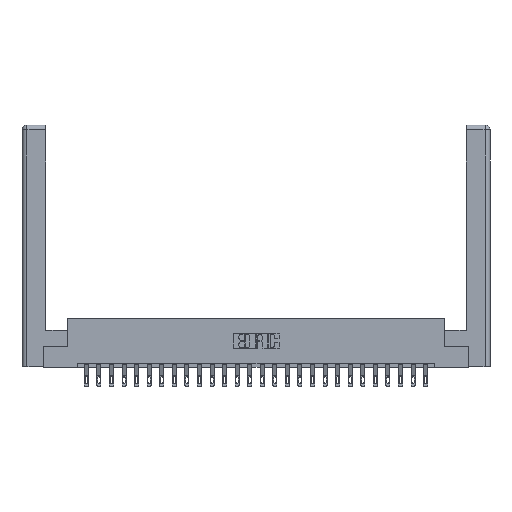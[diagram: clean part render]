
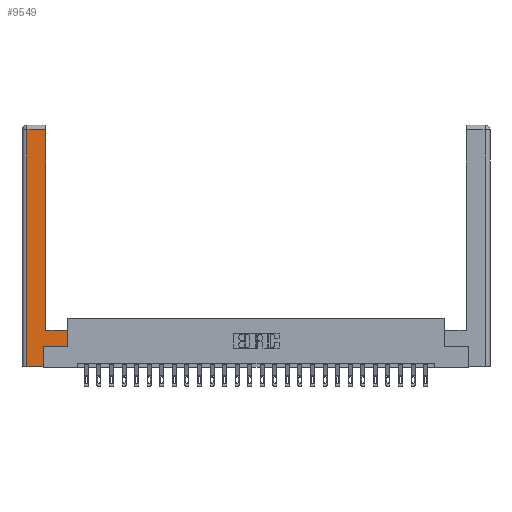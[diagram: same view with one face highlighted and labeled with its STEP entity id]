
A CAD part, top view. The second image highlights one B-rep face of the part: STEP entity #9549.
In plain terms, the highlighted planar face has unit normal (0, 0, 1).
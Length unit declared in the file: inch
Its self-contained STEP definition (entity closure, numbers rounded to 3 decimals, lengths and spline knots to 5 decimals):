
#524 = VECTOR ( 'NONE', #18206, 39.37008 ) ;
#1077 = CARTESIAN_POINT ( 'NONE',  ( 0.295, 0.45, 0. ) ) ;
#1786 = VERTEX_POINT ( 'NONE', #4299 ) ;
#1950 = VECTOR ( 'NONE', #4776, 39.37008 ) ;
#1952 = LINE ( 'NONE', #15213, #2944 ) ;
#2944 = VECTOR ( 'NONE', #9222, 39.37008 ) ;
#3735 = DIRECTION ( 'NONE',  ( 0., -1., 0. ) ) ;
#3939 = DIRECTION ( 'NONE',  ( -1., 0., 0. ) ) ;
#4116 = LINE ( 'NONE', #19426, #13725 ) ;
#4267 = ORIENTED_EDGE ( 'NONE', *, *, #15548, .T. ) ;
#4299 = CARTESIAN_POINT ( 'NONE',  ( 0.0615, 0., 0. ) ) ;
#4776 = DIRECTION ( 'NONE',  ( 0., 1., 0. ) ) ;
#5395 = LINE ( 'NONE', #19114, #13722 ) ;
#6811 = VERTEX_POINT ( 'NONE', #16730 ) ;
#7710 = DIRECTION ( 'NONE',  ( -1., 0., 0. ) ) ;
#8630 = EDGE_CURVE ( 'NONE', #1786, #24178, #4116, .T. ) ;
#8959 = CARTESIAN_POINT ( 'NONE',  ( 0.295, 3., 0. ) ) ;
#9195 = CARTESIAN_POINT ( 'NONE',  ( 0.565, 0.245, 0. ) ) ;
#9222 = DIRECTION ( 'NONE',  ( 1., 0., 0. ) ) ;
#9431 = ORIENTED_EDGE ( 'NONE', *, *, #19889, .T. ) ;
#9549 = ADVANCED_FACE ( 'NONE', ( #22116 ), #11859, .F. ) ;
#9578 = LINE ( 'NONE', #9770, #13397 ) ;
#9770 = CARTESIAN_POINT ( 'NONE',  ( 0.0615, 0., 0. ) ) ;
#10397 = AXIS2_PLACEMENT_3D ( 'NONE', #17906, #26095, #13889 ) ;
#10983 = LINE ( 'NONE', #21126, #1950 ) ;
#11367 = DIRECTION ( 'NONE',  ( 1., 0., 0. ) ) ;
#11859 = PLANE ( 'NONE',  #10397 ) ;
#11881 = EDGE_LOOP ( 'NONE', ( #12309, #22822, #21513, #19605, #4267, #16017, #9431, #15702 ) ) ;
#12309 = ORIENTED_EDGE ( 'NONE', *, *, #19631, .T. ) ;
#12325 = EDGE_CURVE ( 'NONE', #19669, #20694, #1952, .T. ) ;
#13099 = VECTOR ( 'NONE', #3939, 39.37008 ) ;
#13397 = VECTOR ( 'NONE', #3735, 39.37008 ) ;
#13579 = CARTESIAN_POINT ( 'NONE',  ( 0.265, 0.245, 0. ) ) ;
#13644 = EDGE_CURVE ( 'NONE', #21884, #15916, #5395, .T. ) ;
#13722 = VECTOR ( 'NONE', #7710, 39.37008 ) ;
#13725 = VECTOR ( 'NONE', #11367, 39.37008 ) ;
#13889 = DIRECTION ( 'NONE',  ( -1., 0., 0. ) ) ;
#14695 = CARTESIAN_POINT ( 'NONE',  ( 0.0615, 2.94, 0. ) ) ;
#15213 = CARTESIAN_POINT ( 'NONE',  ( 0.565, 0.245, 0. ) ) ;
#15548 = EDGE_CURVE ( 'NONE', #24178, #19669, #10983, .T. ) ;
#15702 = ORIENTED_EDGE ( 'NONE', *, *, #22205, .T. ) ;
#15916 = VERTEX_POINT ( 'NONE', #14695 ) ;
#15961 = LINE ( 'NONE', #8959, #19411 ) ;
#16017 = ORIENTED_EDGE ( 'NONE', *, *, #12325, .T. ) ;
#16587 = LINE ( 'NONE', #18728, #524 ) ;
#16730 = CARTESIAN_POINT ( 'NONE',  ( 0.565, 0.45, 0. ) ) ;
#16834 = VERTEX_POINT ( 'NONE', #1077 ) ;
#17300 = CARTESIAN_POINT ( 'NONE',  ( 0.295, 2.94, 0. ) ) ;
#17906 = CARTESIAN_POINT ( 'NONE',  ( 0., 0., 0. ) ) ;
#18206 = DIRECTION ( 'NONE',  ( 0., 1., 0. ) ) ;
#18529 = EDGE_CURVE ( 'NONE', #15916, #1786, #9578, .T. ) ;
#18728 = CARTESIAN_POINT ( 'NONE',  ( 0.565, 0.45, 0. ) ) ;
#19114 = CARTESIAN_POINT ( 'NONE',  ( 0.0615, 2.94, 0. ) ) ;
#19411 = VECTOR ( 'NONE', #25188, 39.37008 ) ;
#19426 = CARTESIAN_POINT ( 'NONE',  ( 0.265, 0., 0. ) ) ;
#19605 = ORIENTED_EDGE ( 'NONE', *, *, #8630, .T. ) ;
#19631 = EDGE_CURVE ( 'NONE', #16834, #21884, #15961, .T. ) ;
#19669 = VERTEX_POINT ( 'NONE', #13579 ) ;
#19889 = EDGE_CURVE ( 'NONE', #20694, #6811, #16587, .T. ) ;
#20694 = VERTEX_POINT ( 'NONE', #9195 ) ;
#21126 = CARTESIAN_POINT ( 'NONE',  ( 0.265, 0.245, 0. ) ) ;
#21513 = ORIENTED_EDGE ( 'NONE', *, *, #18529, .T. ) ;
#21884 = VERTEX_POINT ( 'NONE', #17300 ) ;
#22116 = FACE_OUTER_BOUND ( 'NONE', #11881, .T. ) ;
#22205 = EDGE_CURVE ( 'NONE', #6811, #16834, #22991, .T. ) ;
#22822 = ORIENTED_EDGE ( 'NONE', *, *, #13644, .T. ) ;
#22991 = LINE ( 'NONE', #26258, #13099 ) ;
#24178 = VERTEX_POINT ( 'NONE', #24684 ) ;
#24684 = CARTESIAN_POINT ( 'NONE',  ( 0.265, 0., 0. ) ) ;
#25188 = DIRECTION ( 'NONE',  ( 0., 1., 0. ) ) ;
#26095 = DIRECTION ( 'NONE',  ( 0., 0., -1. ) ) ;
#26258 = CARTESIAN_POINT ( 'NONE',  ( 0.295, 0.45, 0. ) ) ;
